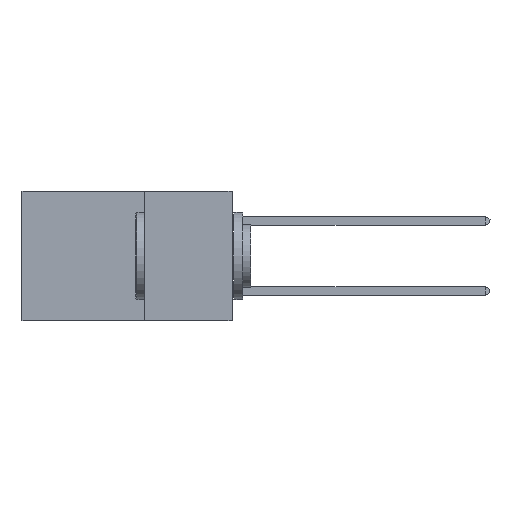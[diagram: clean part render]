
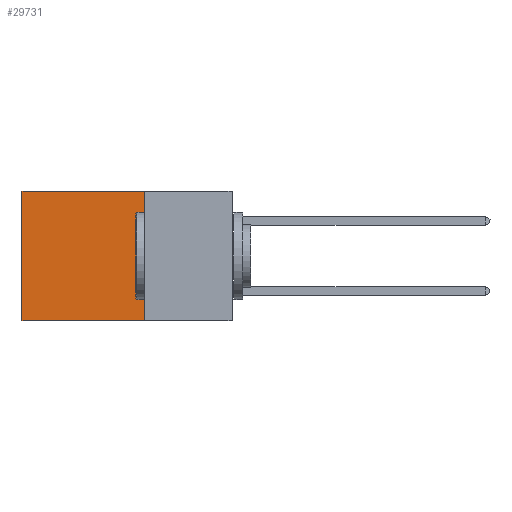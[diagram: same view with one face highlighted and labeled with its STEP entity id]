
A CAD part, left-side view. The second image highlights one B-rep face of the part: STEP entity #29731.
In plain terms, the highlighted planar face has unit normal (-1, 0, 0).
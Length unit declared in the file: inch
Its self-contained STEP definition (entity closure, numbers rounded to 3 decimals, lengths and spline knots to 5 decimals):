
#711 = PLANE ( 'NONE',  #2868 ) ;
#845 = ORIENTED_EDGE ( 'NONE', *, *, #24168, .F. ) ;
#1431 = DIRECTION ( 'NONE',  ( 0., 0., -1. ) ) ;
#1632 = DIRECTION ( 'NONE',  ( 0., 0., -1. ) ) ;
#2868 = AXIS2_PLACEMENT_3D ( 'NONE', #10016, #7737, #1431 ) ;
#5542 = CARTESIAN_POINT ( 'NONE',  ( 0.2875, 0.25, -0.37 ) ) ;
#6806 = ORIENTED_EDGE ( 'NONE', *, *, #39707, .T. ) ;
#7737 = DIRECTION ( 'NONE',  ( 1., 0., 0. ) ) ;
#8825 = VECTOR ( 'NONE', #1632, 39.37008 ) ;
#10016 = CARTESIAN_POINT ( 'NONE',  ( 0.2875, 0.25, 0. ) ) ;
#12020 = VERTEX_POINT ( 'NONE', #32983 ) ;
#12140 = VECTOR ( 'NONE', #36406, 39.37008 ) ;
#14767 = CARTESIAN_POINT ( 'NONE',  ( 0.2875, 0.25, -0.37 ) ) ;
#15287 = VERTEX_POINT ( 'NONE', #36701 ) ;
#19379 = VECTOR ( 'NONE', #20625, 39.37008 ) ;
#20625 = DIRECTION ( 'NONE',  ( 0., 1., 0. ) ) ;
#20746 = CARTESIAN_POINT ( 'NONE',  ( 0.2875, 0.25, 0. ) ) ;
#21511 = VECTOR ( 'NONE', #39431, 39.37008 ) ;
#24168 = EDGE_CURVE ( 'NONE', #31015, #30679, #34402, .T. ) ;
#27675 = LINE ( 'NONE', #20746, #19379 ) ;
#29415 = CARTESIAN_POINT ( 'NONE',  ( 0.2875, 0.6, -0.37 ) ) ;
#29731 = ADVANCED_FACE ( 'NONE', ( #39575 ), #711, .F. ) ;
#30574 = CARTESIAN_POINT ( 'NONE',  ( 0.2875, 0.25, 0. ) ) ;
#30679 = VERTEX_POINT ( 'NONE', #29415 ) ;
#31015 = VERTEX_POINT ( 'NONE', #5542 ) ;
#31592 = EDGE_CURVE ( 'NONE', #12020, #31015, #35497, .T. ) ;
#31600 = LINE ( 'NONE', #39176, #8825 ) ;
#32274 = EDGE_LOOP ( 'NONE', ( #36664, #845, #34981, #6806 ) ) ;
#32983 = CARTESIAN_POINT ( 'NONE',  ( 0.2875, 0.25, 0. ) ) ;
#34402 = LINE ( 'NONE', #14767, #12140 ) ;
#34981 = ORIENTED_EDGE ( 'NONE', *, *, #31592, .F. ) ;
#35497 = LINE ( 'NONE', #30574, #21511 ) ;
#36406 = DIRECTION ( 'NONE',  ( 0., 1., 0. ) ) ;
#36664 = ORIENTED_EDGE ( 'NONE', *, *, #38451, .T. ) ;
#36701 = CARTESIAN_POINT ( 'NONE',  ( 0.2875, 0.6, 0. ) ) ;
#38451 = EDGE_CURVE ( 'NONE', #15287, #30679, #31600, .T. ) ;
#39176 = CARTESIAN_POINT ( 'NONE',  ( 0.2875, 0.6, 0. ) ) ;
#39431 = DIRECTION ( 'NONE',  ( 0., 0., -1. ) ) ;
#39575 = FACE_OUTER_BOUND ( 'NONE', #32274, .T. ) ;
#39707 = EDGE_CURVE ( 'NONE', #12020, #15287, #27675, .T. ) ;
